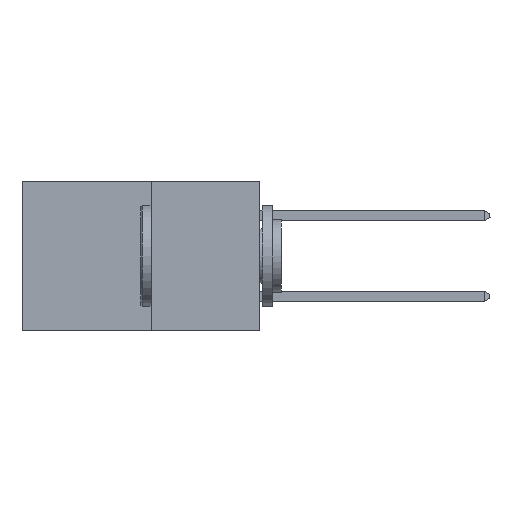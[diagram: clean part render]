
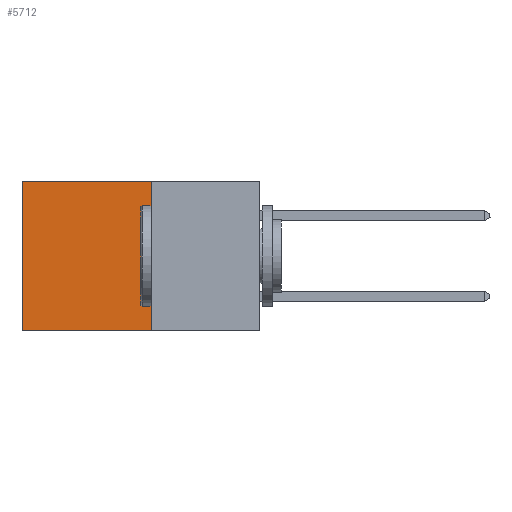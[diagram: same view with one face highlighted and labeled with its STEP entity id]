
A CAD part, left-side view. The second image highlights one B-rep face of the part: STEP entity #5712.
In plain terms, the highlighted planar face has unit normal (-1, 0, 0).
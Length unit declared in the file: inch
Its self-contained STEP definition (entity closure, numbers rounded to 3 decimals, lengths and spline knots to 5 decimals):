
#115 = VERTEX_POINT ( 'NONE', #2484 ) ;
#238 = EDGE_CURVE ( 'NONE', #115, #2298, #1355, .T. ) ;
#290 = EDGE_CURVE ( 'NONE', #2298, #312, #2965, .T. ) ;
#312 = VERTEX_POINT ( 'NONE', #322 ) ;
#322 = CARTESIAN_POINT ( 'NONE',  ( 0.277, 0.59, -0.37 ) ) ;
#618 = DIRECTION ( 'NONE',  ( 0., 1., 0. ) ) ;
#757 = CARTESIAN_POINT ( 'NONE',  ( 0.277, 0.27, 0. ) ) ;
#1007 = FACE_OUTER_BOUND ( 'NONE', #3934, .T. ) ;
#1266 = EDGE_CURVE ( 'NONE', #3027, #312, #7308, .T. ) ;
#1355 = LINE ( 'NONE', #8179, #8403 ) ;
#1791 = DIRECTION ( 'NONE',  ( 0., 0., -1. ) ) ;
#2298 = VERTEX_POINT ( 'NONE', #4208 ) ;
#2484 = CARTESIAN_POINT ( 'NONE',  ( 0.277, 0.27, 0. ) ) ;
#2965 = LINE ( 'NONE', #4776, #4161 ) ;
#3027 = VERTEX_POINT ( 'NONE', #5906 ) ;
#3721 = VECTOR ( 'NONE', #1791, 39.37008 ) ;
#3890 = CARTESIAN_POINT ( 'NONE',  ( 0.277, 0.59, -0.37 ) ) ;
#3934 = EDGE_LOOP ( 'NONE', ( #6297, #6288, #6338, #6456 ) ) ;
#4139 = LINE ( 'NONE', #757, #7533 ) ;
#4161 = VECTOR ( 'NONE', #8503, 39.37008 ) ;
#4208 = CARTESIAN_POINT ( 'NONE',  ( 0.277, 0.27, -0.37 ) ) ;
#4776 = CARTESIAN_POINT ( 'NONE',  ( 0.277, 0.27, -0.37 ) ) ;
#5712 = ADVANCED_FACE ( 'NONE', ( #1007 ), #7656, .F. ) ;
#5906 = CARTESIAN_POINT ( 'NONE',  ( 0.277, 0.59, 0. ) ) ;
#6288 = ORIENTED_EDGE ( 'NONE', *, *, #290, .F. ) ;
#6297 = ORIENTED_EDGE ( 'NONE', *, *, #1266, .T. ) ;
#6338 = ORIENTED_EDGE ( 'NONE', *, *, #238, .F. ) ;
#6456 = ORIENTED_EDGE ( 'NONE', *, *, #7523, .T. ) ;
#7131 = AXIS2_PLACEMENT_3D ( 'NONE', #7932, #8445, #7592 ) ;
#7308 = LINE ( 'NONE', #3890, #3721 ) ;
#7523 = EDGE_CURVE ( 'NONE', #115, #3027, #4139, .T. ) ;
#7533 = VECTOR ( 'NONE', #618, 39.37008 ) ;
#7592 = DIRECTION ( 'NONE',  ( 0., 0., -1. ) ) ;
#7656 = PLANE ( 'NONE',  #7131 ) ;
#7932 = CARTESIAN_POINT ( 'NONE',  ( 0.277, 0.27, -0.37 ) ) ;
#8057 = DIRECTION ( 'NONE',  ( 0., 0., -1. ) ) ;
#8179 = CARTESIAN_POINT ( 'NONE',  ( 0.277, 0.27, -0.37 ) ) ;
#8403 = VECTOR ( 'NONE', #8057, 39.37008 ) ;
#8445 = DIRECTION ( 'NONE',  ( 1., 0., 0. ) ) ;
#8503 = DIRECTION ( 'NONE',  ( 0., 1., 0. ) ) ;
